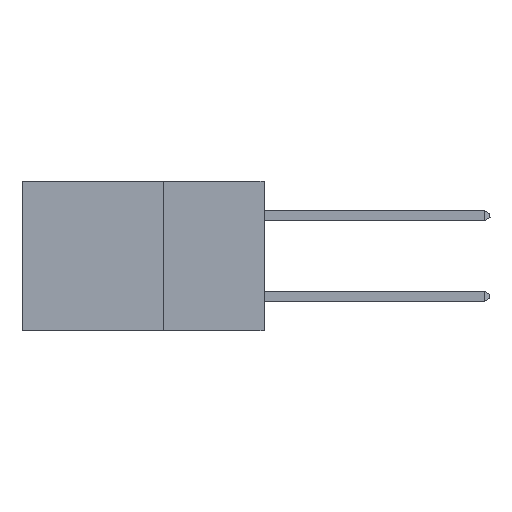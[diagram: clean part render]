
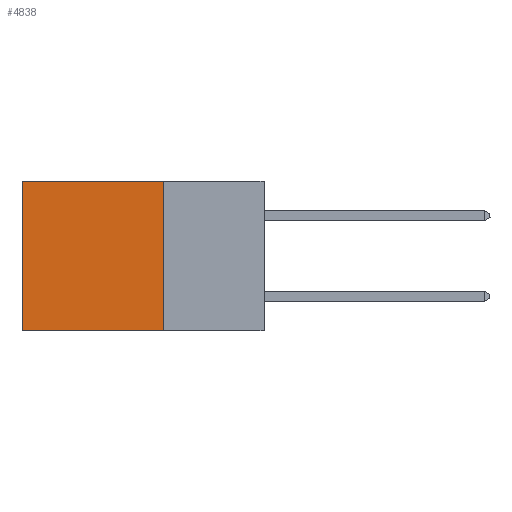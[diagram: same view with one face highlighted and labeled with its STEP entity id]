
A CAD part, left-side view. The second image highlights one B-rep face of the part: STEP entity #4838.
In plain terms, the highlighted planar face has unit normal (-1, 0, 0).
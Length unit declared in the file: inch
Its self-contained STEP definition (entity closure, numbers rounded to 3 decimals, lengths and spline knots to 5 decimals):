
#78 = CARTESIAN_POINT ( 'NONE',  ( 0.298, 0.6, 0. ) ) ;
#345 = CARTESIAN_POINT ( 'NONE',  ( 0.298, 0.25, 0. ) ) ;
#736 = CARTESIAN_POINT ( 'NONE',  ( 0.298, 0.25, 0. ) ) ;
#806 = VECTOR ( 'NONE', #13535, 39.37008 ) ;
#807 = CARTESIAN_POINT ( 'NONE',  ( 0.298, 0.25, -0.37 ) ) ;
#820 = VERTEX_POINT ( 'NONE', #11375 ) ;
#1130 = ORIENTED_EDGE ( 'NONE', *, *, #14750, .T. ) ;
#1913 = LINE ( 'NONE', #345, #12271 ) ;
#1975 = DIRECTION ( 'NONE',  ( 1., 0., 0. ) ) ;
#1982 = EDGE_CURVE ( 'NONE', #820, #8150, #3174, .T. ) ;
#3174 = LINE ( 'NONE', #807, #806 ) ;
#4838 = ADVANCED_FACE ( 'NONE', ( #8365 ), #8397, .F. ) ;
#6157 = CARTESIAN_POINT ( 'NONE',  ( 0.298, 0.6, -0.37 ) ) ;
#8150 = VERTEX_POINT ( 'NONE', #6157 ) ;
#8237 = CARTESIAN_POINT ( 'NONE',  ( 0.298, 0.6, 0. ) ) ;
#8365 = FACE_OUTER_BOUND ( 'NONE', #15749, .T. ) ;
#8397 = PLANE ( 'NONE',  #9818 ) ;
#8901 = LINE ( 'NONE', #8237, #13693 ) ;
#9076 = ORIENTED_EDGE ( 'NONE', *, *, #14475, .F. ) ;
#9227 = DIRECTION ( 'NONE',  ( 0., 0., -1. ) ) ;
#9373 = ORIENTED_EDGE ( 'NONE', *, *, #1982, .F. ) ;
#9571 = CARTESIAN_POINT ( 'NONE',  ( 0.298, 0.25, 0. ) ) ;
#9818 = AXIS2_PLACEMENT_3D ( 'NONE', #9571, #1975, #10922 ) ;
#10452 = VECTOR ( 'NONE', #10893, 39.37008 ) ;
#10561 = VERTEX_POINT ( 'NONE', #78 ) ;
#10893 = DIRECTION ( 'NONE',  ( 0., 1., 0. ) ) ;
#10922 = DIRECTION ( 'NONE',  ( 0., 0., -1. ) ) ;
#11375 = CARTESIAN_POINT ( 'NONE',  ( 0.298, 0.25, -0.37 ) ) ;
#11550 = EDGE_CURVE ( 'NONE', #10561, #8150, #8901, .T. ) ;
#11697 = CARTESIAN_POINT ( 'NONE',  ( 0.298, 0.25, 0. ) ) ;
#11887 = LINE ( 'NONE', #736, #10452 ) ;
#12054 = DIRECTION ( 'NONE',  ( 0., 0., -1. ) ) ;
#12271 = VECTOR ( 'NONE', #9227, 39.37008 ) ;
#13395 = ORIENTED_EDGE ( 'NONE', *, *, #11550, .T. ) ;
#13535 = DIRECTION ( 'NONE',  ( 0., 1., 0. ) ) ;
#13693 = VECTOR ( 'NONE', #12054, 39.37008 ) ;
#14475 = EDGE_CURVE ( 'NONE', #15152, #820, #1913, .T. ) ;
#14750 = EDGE_CURVE ( 'NONE', #15152, #10561, #11887, .T. ) ;
#15152 = VERTEX_POINT ( 'NONE', #11697 ) ;
#15749 = EDGE_LOOP ( 'NONE', ( #13395, #9373, #9076, #1130 ) ) ;
